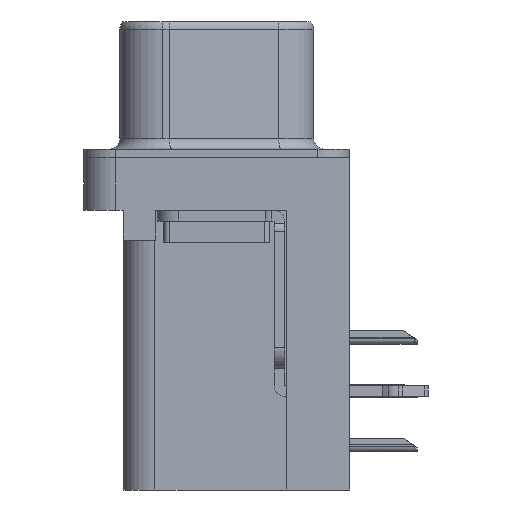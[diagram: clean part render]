
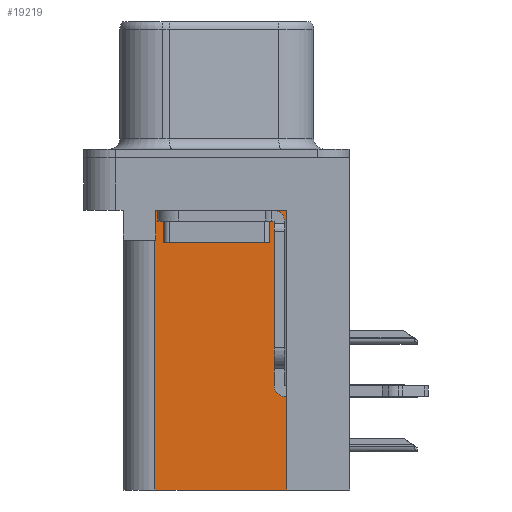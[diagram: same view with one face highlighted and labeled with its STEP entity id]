
A CAD part, left-side view. The second image highlights one B-rep face of the part: STEP entity #19219.
In plain terms, the highlighted planar face has unit normal (-1, 0, 0).
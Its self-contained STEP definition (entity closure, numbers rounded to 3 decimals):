
#463 = CARTESIAN_POINT ( 'NONE',  ( 3.7, -3.295, -15.7 ) ) ;
#527 = DIRECTION ( 'NONE',  ( 0., 1., 0. ) ) ;
#796 = DIRECTION ( 'NONE',  ( 0., 1., 0. ) ) ;
#1288 = EDGE_CURVE ( 'NONE', #7610, #27853, #21472, .T. ) ;
#1885 = DIRECTION ( 'NONE',  ( 0., 0., -1. ) ) ;
#2792 = CARTESIAN_POINT ( 'NONE',  ( 3.7, 2.925, -15.7 ) ) ;
#2828 = LINE ( 'NONE', #12609, #8456 ) ;
#2999 = VECTOR ( 'NONE', #6599, 1000. ) ;
#3261 = VECTOR ( 'NONE', #527, 1000. ) ;
#3554 = LINE ( 'NONE', #2792, #21270 ) ;
#4058 = LINE ( 'NONE', #28452, #3261 ) ;
#4364 = CARTESIAN_POINT ( 'NONE',  ( 3.7, -3.295, -15.7 ) ) ;
#5071 = EDGE_CURVE ( 'NONE', #27648, #25995, #2828, .T. ) ;
#5191 = CARTESIAN_POINT ( 'NONE',  ( 3.7, -3.295, -15.7 ) ) ;
#5312 = DIRECTION ( 'NONE',  ( 0., 0., 1. ) ) ;
#5486 = DIRECTION ( 'NONE',  ( 1., 0., 0. ) ) ;
#6599 = DIRECTION ( 'NONE',  ( 0., 1., 0. ) ) ;
#7610 = VERTEX_POINT ( 'NONE', #4364 ) ;
#7889 = LINE ( 'NONE', #13583, #19251 ) ;
#8456 = VECTOR ( 'NONE', #796, 1000. ) ;
#8601 = CARTESIAN_POINT ( 'NONE',  ( 3.7, -3.295, -2.5 ) ) ;
#9391 = ORIENTED_EDGE ( 'NONE', *, *, #29484, .T. ) ;
#10039 = PLANE ( 'NONE',  #29180 ) ;
#10069 = ORIENTED_EDGE ( 'NONE', *, *, #18484, .T. ) ;
#10988 = CARTESIAN_POINT ( 'NONE',  ( 3.7, 2.895, -2.5 ) ) ;
#11438 = ORIENTED_EDGE ( 'NONE', *, *, #1288, .F. ) ;
#12609 = CARTESIAN_POINT ( 'NONE',  ( 3.7, -3.295, -2.5 ) ) ;
#12687 = LINE ( 'NONE', #27944, #23419 ) ;
#12991 = FACE_OUTER_BOUND ( 'NONE', #13141, .T. ) ;
#13141 = EDGE_LOOP ( 'NONE', ( #28725, #25956, #9391, #13176, #11438, #10069 ) ) ;
#13176 = ORIENTED_EDGE ( 'NONE', *, *, #18592, .F. ) ;
#13370 = VERTEX_POINT ( 'NONE', #21590 ) ;
#13583 = CARTESIAN_POINT ( 'NONE',  ( 3.7, 2.895, -3.9 ) ) ;
#18484 = EDGE_CURVE ( 'NONE', #7610, #27648, #12687, .T. ) ;
#18592 = EDGE_CURVE ( 'NONE', #27853, #20596, #3554, .T. ) ;
#19219 = ADVANCED_FACE ( 'NONE', ( #12991 ), #10039, .F. ) ;
#19251 = VECTOR ( 'NONE', #1885, 1000. ) ;
#20596 = VERTEX_POINT ( 'NONE', #23508 ) ;
#21270 = VECTOR ( 'NONE', #5312, 1000. ) ;
#21472 = LINE ( 'NONE', #5191, #2999 ) ;
#21479 = DIRECTION ( 'NONE',  ( 0., 0., -1. ) ) ;
#21590 = CARTESIAN_POINT ( 'NONE',  ( 3.7, 2.895, -3.9 ) ) ;
#22956 = CARTESIAN_POINT ( 'NONE',  ( 3.7, 2.925, -15.7 ) ) ;
#23233 = DIRECTION ( 'NONE',  ( 0., 0., 1. ) ) ;
#23419 = VECTOR ( 'NONE', #23233, 1000. ) ;
#23508 = CARTESIAN_POINT ( 'NONE',  ( 3.7, 2.925, -3.9 ) ) ;
#25956 = ORIENTED_EDGE ( 'NONE', *, *, #26792, .T. ) ;
#25995 = VERTEX_POINT ( 'NONE', #10988 ) ;
#26792 = EDGE_CURVE ( 'NONE', #25995, #13370, #7889, .T. ) ;
#27648 = VERTEX_POINT ( 'NONE', #8601 ) ;
#27853 = VERTEX_POINT ( 'NONE', #22956 ) ;
#27944 = CARTESIAN_POINT ( 'NONE',  ( 3.7, -3.295, -15.7 ) ) ;
#28452 = CARTESIAN_POINT ( 'NONE',  ( 3.7, 0., -3.9 ) ) ;
#28725 = ORIENTED_EDGE ( 'NONE', *, *, #5071, .T. ) ;
#29180 = AXIS2_PLACEMENT_3D ( 'NONE', #463, #5486, #21479 ) ;
#29484 = EDGE_CURVE ( 'NONE', #13370, #20596, #4058, .T. ) ;
